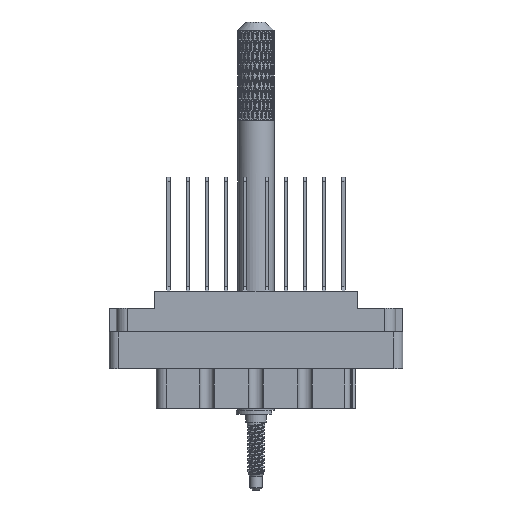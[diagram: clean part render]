
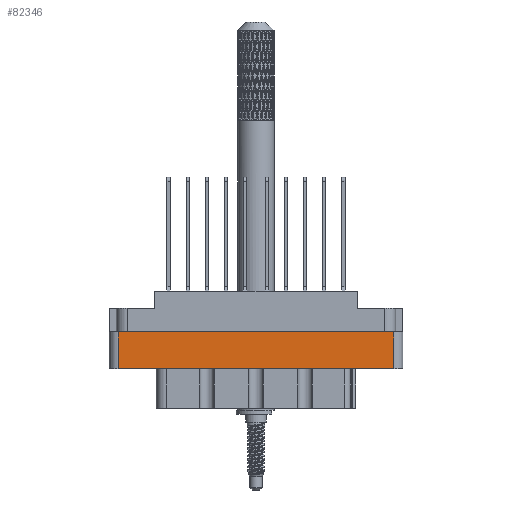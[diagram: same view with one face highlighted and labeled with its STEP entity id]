
A CAD part, front view. The second image highlights one B-rep face of the part: STEP entity #82346.
In plain terms, the highlighted planar face has unit normal (0, -1, 0).
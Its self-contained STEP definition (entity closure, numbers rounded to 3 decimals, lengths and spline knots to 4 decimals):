
#2847 = LINE ( 'NONE', #6599, #64645 ) ;
#6223 = DIRECTION ( 'NONE',  ( 0., -1., 0. ) ) ;
#6599 = CARTESIAN_POINT ( 'NONE',  ( -0.938, -0.438, -0.798 ) ) ;
#6748 = CARTESIAN_POINT ( 'NONE',  ( -0.938, -0.438, -0.529 ) ) ;
#12188 = ORIENTED_EDGE ( 'NONE', *, *, #22007, .F. ) ;
#13671 = DIRECTION ( 'NONE',  ( 0., 0., -1. ) ) ;
#15428 = CARTESIAN_POINT ( 'NONE',  ( 0., -0.438, -0.277 ) ) ;
#16132 = DIRECTION ( 'NONE',  ( 0., 0., 1. ) ) ;
#17707 = VERTEX_POINT ( 'NONE', #61909 ) ;
#18465 = VECTOR ( 'NONE', #48011, 39.3701 ) ;
#18940 = VECTOR ( 'NONE', #16132, 39.3701 ) ;
#22007 = EDGE_CURVE ( 'NONE', #81887, #31494, #45380, .T. ) ;
#24391 = CARTESIAN_POINT ( 'NONE',  ( 0., -0.438, -0.529 ) ) ;
#28073 = AXIS2_PLACEMENT_3D ( 'NONE', #53822, #6223, #13671 ) ;
#31494 = VERTEX_POINT ( 'NONE', #54791 ) ;
#33600 = LINE ( 'NONE', #24391, #18465 ) ;
#34978 = CARTESIAN_POINT ( 'NONE',  ( -0.938, -0.438, -0.277 ) ) ;
#45380 = LINE ( 'NONE', #15428, #93345 ) ;
#48011 = DIRECTION ( 'NONE',  ( -1., 0., 0. ) ) ;
#53822 = CARTESIAN_POINT ( 'NONE',  ( -1., -0.438, -0.798 ) ) ;
#54791 = CARTESIAN_POINT ( 'NONE',  ( 0.938, -0.438, -0.277 ) ) ;
#60965 = FACE_OUTER_BOUND ( 'NONE', #83867, .T. ) ;
#61130 = EDGE_CURVE ( 'NONE', #17707, #85917, #33600, .T. ) ;
#61238 = PLANE ( 'NONE',  #28073 ) ;
#61909 = CARTESIAN_POINT ( 'NONE',  ( 0.938, -0.438, -0.529 ) ) ;
#64262 = EDGE_CURVE ( 'NONE', #81887, #85917, #2847, .T. ) ;
#64645 = VECTOR ( 'NONE', #102896, 39.3701 ) ;
#70401 = DIRECTION ( 'NONE',  ( 1., 0., 0. ) ) ;
#72158 = CARTESIAN_POINT ( 'NONE',  ( 0.938, -0.438, -0.798 ) ) ;
#77001 = LINE ( 'NONE', #72158, #18940 ) ;
#81887 = VERTEX_POINT ( 'NONE', #34978 ) ;
#82346 = ADVANCED_FACE ( 'NONE', ( #60965 ), #61238, .T. ) ;
#83156 = ORIENTED_EDGE ( 'NONE', *, *, #61130, .F. ) ;
#83867 = EDGE_LOOP ( 'NONE', ( #12188, #102319, #83156, #98364 ) ) ;
#85917 = VERTEX_POINT ( 'NONE', #6748 ) ;
#86974 = EDGE_CURVE ( 'NONE', #17707, #31494, #77001, .T. ) ;
#93345 = VECTOR ( 'NONE', #70401, 39.3701 ) ;
#98364 = ORIENTED_EDGE ( 'NONE', *, *, #86974, .T. ) ;
#102319 = ORIENTED_EDGE ( 'NONE', *, *, #64262, .T. ) ;
#102896 = DIRECTION ( 'NONE',  ( 0., 0., -1. ) ) ;
